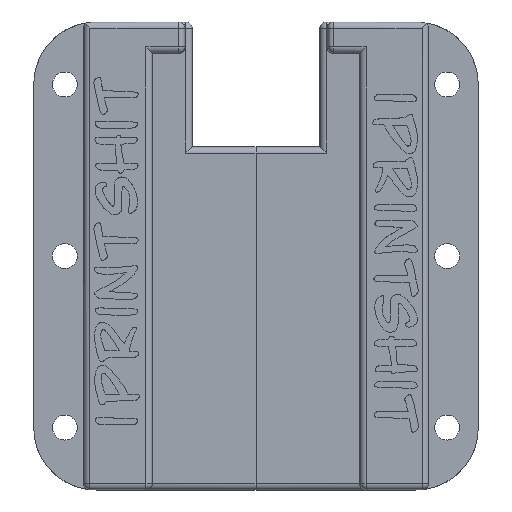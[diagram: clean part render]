
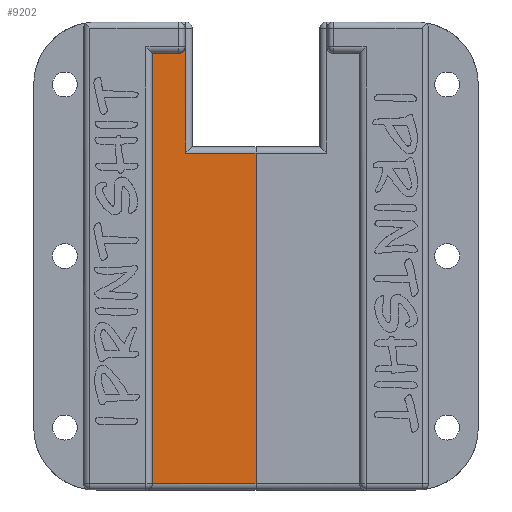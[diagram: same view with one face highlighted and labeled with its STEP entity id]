
A CAD part, top view. The second image highlights one B-rep face of the part: STEP entity #9202.
In plain terms, the highlighted planar face has unit normal (0, 0, 1).
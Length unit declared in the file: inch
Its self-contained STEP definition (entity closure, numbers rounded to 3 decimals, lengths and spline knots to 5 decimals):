
#105=ELLIPSE('',#9559,0.05,0.05);
#255=PLANE('',#9599);
#562=FACE_OUTER_BOUND('',#1104,.T.);
#1104=EDGE_LOOP('',(#7114,#7115,#7116,#7117,#7118,#7119,#7120,#7121,#7122));
#1665=LINE('',#14458,#2297);
#1674=LINE('',#14503,#2306);
#1698=LINE('',#14583,#2330);
#1706=LINE('',#14611,#2338);
#1707=LINE('',#14613,#2339);
#1708=LINE('',#14615,#2340);
#1709=LINE('',#14617,#2341);
#1710=LINE('',#14618,#2342);
#2297=VECTOR('',#10108,39.37008);
#2306=VECTOR('',#10157,39.37008);
#2330=VECTOR('',#10239,0.3937);
#2338=VECTOR('',#10273,39.37008);
#2339=VECTOR('',#10274,39.37008);
#2340=VECTOR('',#10275,39.37008);
#2341=VECTOR('',#10276,39.37008);
#2342=VECTOR('',#10277,39.37008);
#3788=VERTEX_POINT('',#14455);
#3789=VERTEX_POINT('',#14457);
#3801=VERTEX_POINT('',#14501);
#3802=VERTEX_POINT('',#14505);
#3827=VERTEX_POINT('',#14580);
#3828=VERTEX_POINT('',#14582);
#3836=VERTEX_POINT('',#14612);
#3837=VERTEX_POINT('',#14614);
#3838=VERTEX_POINT('',#14616);
#4935=EDGE_CURVE('',#3789,#3788,#1665,.T.);
#4956=EDGE_CURVE('',#3801,#3788,#1674,.T.);
#4957=EDGE_CURVE('',#3789,#3802,#105,.T.);
#4995=EDGE_CURVE('',#3827,#3828,#1698,.T.);
#5010=EDGE_CURVE('',#3828,#3801,#1706,.T.);
#5011=EDGE_CURVE('',#3836,#3827,#1707,.T.);
#5012=EDGE_CURVE('',#3837,#3836,#1708,.T.);
#5013=EDGE_CURVE('',#3838,#3837,#1709,.T.);
#5014=EDGE_CURVE('',#3802,#3838,#1710,.T.);
#7114=ORIENTED_EDGE('',*,*,#4956,.F.);
#7115=ORIENTED_EDGE('',*,*,#5010,.F.);
#7116=ORIENTED_EDGE('',*,*,#4995,.F.);
#7117=ORIENTED_EDGE('',*,*,#5011,.F.);
#7118=ORIENTED_EDGE('',*,*,#5012,.F.);
#7119=ORIENTED_EDGE('',*,*,#5013,.F.);
#7120=ORIENTED_EDGE('',*,*,#5014,.F.);
#7121=ORIENTED_EDGE('',*,*,#4957,.F.);
#7122=ORIENTED_EDGE('',*,*,#4935,.T.);
#9202=ADVANCED_FACE('',(#562),#255,.T.);
#9559=AXIS2_PLACEMENT_3D('',#14506,#10160,#10161);
#9599=AXIS2_PLACEMENT_3D('',#14610,#10271,#10272);
#10108=DIRECTION('',(-1.,0.,0.));
#10157=DIRECTION('',(0.,1.,0.));
#10160=DIRECTION('center_axis',(0.,0.,1.));
#10161=DIRECTION('ref_axis',(1.,0.,0.));
#10239=DIRECTION('',(0.,-1.,0.));
#10271=DIRECTION('center_axis',(0.,0.,1.));
#10272=DIRECTION('ref_axis',(0.,1.,0.));
#10273=DIRECTION('',(-1.,0.,0.));
#10274=DIRECTION('',(1.,0.,0.));
#10275=DIRECTION('',(0.,-1.,0.));
#10276=DIRECTION('',(1.,0.,0.));
#10277=DIRECTION('',(0.,1.,0.));
#14455=CARTESIAN_POINT('',(-1.11438,-0.65,0.4));
#14457=CARTESIAN_POINT('',(-0.89938,-0.65,0.4));
#14458=CARTESIAN_POINT('',(-1.05438,-0.65,0.4));
#14501=CARTESIAN_POINT('',(-1.11438,-4.1,0.4));
#14503=CARTESIAN_POINT('',(-1.11438,-4.83712,0.4));
#14505=CARTESIAN_POINT('',(-0.84938,-0.6,0.4));
#14506=CARTESIAN_POINT('Origin',(-0.89938,-0.6,
0.4));
#14580=CARTESIAN_POINT('',(-0.28219,-1.45,0.4));
#14582=CARTESIAN_POINT('',(-0.28219,-4.1,0.4));
#14583=CARTESIAN_POINT('',(-0.28219,-3.15255,0.4));
#14610=CARTESIAN_POINT('Origin',(-0.56437,-4.15,0.4));
#14611=CARTESIAN_POINT('',(-1.11438,-4.1,0.4));
#14612=CARTESIAN_POINT('',(-0.84438,-1.45,0.4));
#14613=CARTESIAN_POINT('',(-0.56438,-1.45,0.4));
#14614=CARTESIAN_POINT('',(-0.84438,-0.45,0.4));
#14615=CARTESIAN_POINT('',(-0.84438,-4.15,0.4));
#14616=CARTESIAN_POINT('',(-0.84938,-0.45,0.4));
#14617=CARTESIAN_POINT('',(-0.56438,-0.45,0.4));
#14618=CARTESIAN_POINT('',(-0.84938,-1.05376,0.4));
